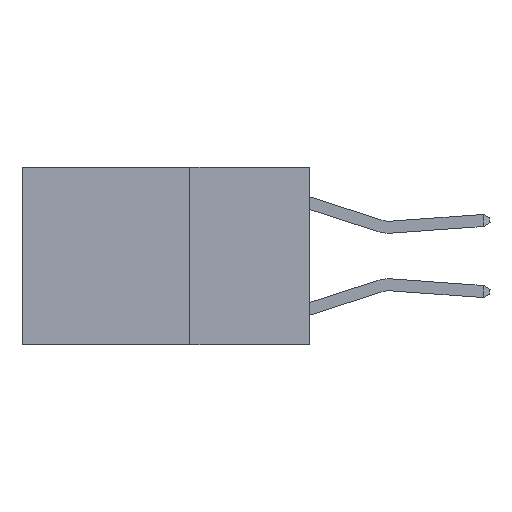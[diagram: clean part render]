
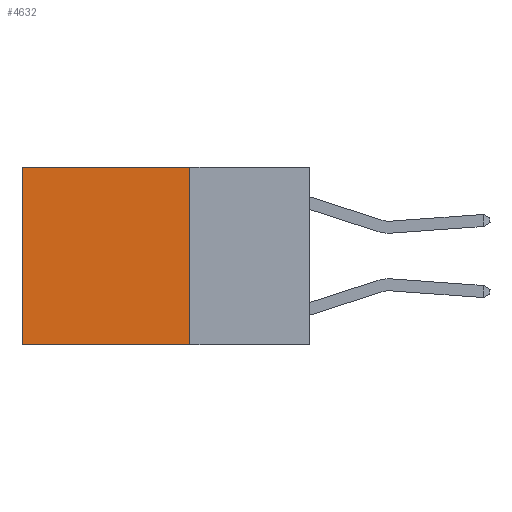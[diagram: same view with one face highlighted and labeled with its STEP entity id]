
A CAD part, left-side view. The second image highlights one B-rep face of the part: STEP entity #4632.
In plain terms, the highlighted planar face has unit normal (-1, 0, 0).
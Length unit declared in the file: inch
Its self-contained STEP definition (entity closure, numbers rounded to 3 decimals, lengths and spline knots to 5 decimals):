
#220 = LINE ( 'NONE', #10553, #8285 ) ;
#286 = CARTESIAN_POINT ( 'NONE',  ( 0.2625, 0.6, 0. ) ) ;
#1161 = CARTESIAN_POINT ( 'NONE',  ( 0.2625, 0.25, 0. ) ) ;
#1201 = CARTESIAN_POINT ( 'NONE',  ( 0.2625, 0.25, -0.37 ) ) ;
#1215 = CARTESIAN_POINT ( 'NONE',  ( 0.2625, 0.6, -0.37 ) ) ;
#1290 = CARTESIAN_POINT ( 'NONE',  ( 0.2625, 0.6, 0. ) ) ;
#1311 = EDGE_CURVE ( 'NONE', #6531, #5853, #9613, .T. ) ;
#2374 = ORIENTED_EDGE ( 'NONE', *, *, #11847, .F. ) ;
#2495 = DIRECTION ( 'NONE',  ( 0., 0., -1. ) ) ;
#2703 = ORIENTED_EDGE ( 'NONE', *, *, #1311, .F. ) ;
#3131 = DIRECTION ( 'NONE',  ( 1., 0., 0. ) ) ;
#4093 = FACE_OUTER_BOUND ( 'NONE', #6499, .T. ) ;
#4467 = AXIS2_PLACEMENT_3D ( 'NONE', #1161, #3131, #5130 ) ;
#4529 = CARTESIAN_POINT ( 'NONE',  ( 0.2625, 0.25, 0. ) ) ;
#4632 = ADVANCED_FACE ( 'NONE', ( #4093 ), #11308, .F. ) ;
#5130 = DIRECTION ( 'NONE',  ( 0., 0., -1. ) ) ;
#5632 = VECTOR ( 'NONE', #2495, 39.37008 ) ;
#5853 = VERTEX_POINT ( 'NONE', #1201 ) ;
#6384 = VECTOR ( 'NONE', #11517, 39.37008 ) ;
#6395 = LINE ( 'NONE', #1290, #8711 ) ;
#6499 = EDGE_LOOP ( 'NONE', ( #11393, #2374, #2703, #10928 ) ) ;
#6531 = VERTEX_POINT ( 'NONE', #9877 ) ;
#6920 = EDGE_CURVE ( 'NONE', #6531, #11454, #220, .T. ) ;
#8285 = VECTOR ( 'NONE', #10438, 39.37008 ) ;
#8442 = DIRECTION ( 'NONE',  ( 0., 0., -1. ) ) ;
#8711 = VECTOR ( 'NONE', #8442, 39.37008 ) ;
#8716 = VERTEX_POINT ( 'NONE', #1215 ) ;
#8851 = EDGE_CURVE ( 'NONE', #11454, #8716, #6395, .T. ) ;
#9613 = LINE ( 'NONE', #4529, #5632 ) ;
#9663 = CARTESIAN_POINT ( 'NONE',  ( 0.2625, 0.25, -0.37 ) ) ;
#9877 = CARTESIAN_POINT ( 'NONE',  ( 0.2625, 0.25, 0. ) ) ;
#10438 = DIRECTION ( 'NONE',  ( 0., 1., 0. ) ) ;
#10553 = CARTESIAN_POINT ( 'NONE',  ( 0.2625, 0.25, 0. ) ) ;
#10928 = ORIENTED_EDGE ( 'NONE', *, *, #6920, .T. ) ;
#11308 = PLANE ( 'NONE',  #4467 ) ;
#11393 = ORIENTED_EDGE ( 'NONE', *, *, #8851, .T. ) ;
#11454 = VERTEX_POINT ( 'NONE', #286 ) ;
#11517 = DIRECTION ( 'NONE',  ( 0., 1., 0. ) ) ;
#11636 = LINE ( 'NONE', #9663, #6384 ) ;
#11847 = EDGE_CURVE ( 'NONE', #5853, #8716, #11636, .T. ) ;
